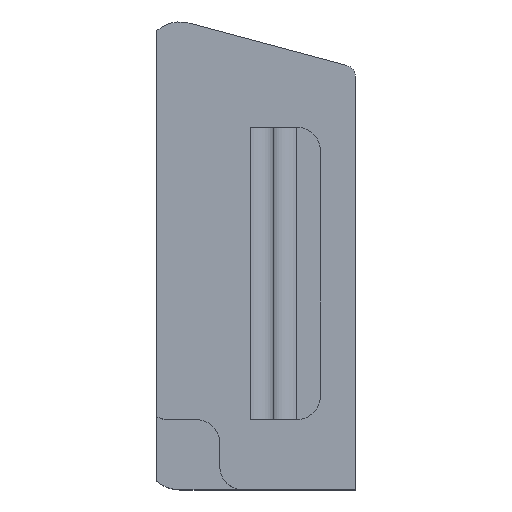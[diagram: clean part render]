
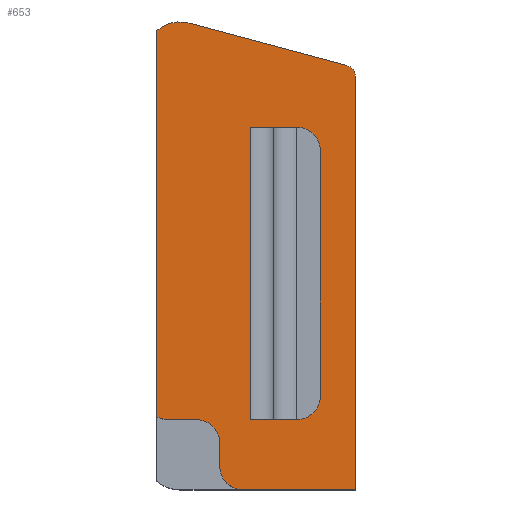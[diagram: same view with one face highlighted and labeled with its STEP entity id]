
A CAD part, top view. The second image highlights one B-rep face of the part: STEP entity #653.
In plain terms, the highlighted planar face has unit normal (0, 0, 1).
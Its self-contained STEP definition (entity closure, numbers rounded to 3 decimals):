
#122=CARTESIAN_POINT('',(-2.0,-30.732,8.0));
#123=VERTEX_POINT('',#122);
#130=CARTESIAN_POINT('',(-2.0,2.236,8.0));
#131=VERTEX_POINT('',#130);
#132=CARTESIAN_POINT('',(-2.0,2.236,8.0));
#133=DIRECTION('',(0.0,-1.0,0.0));
#134=VECTOR('',#133,32.968);
#135=LINE('',#132,#134);
#136=EDGE_CURVE('',#131,#123,#135,.T.);
#320=CARTESIAN_POINT('',(10.,-31.0,8.0));
#321=VERTEX_POINT('',#320);
#328=CARTESIAN_POINT('',(12.,-29.0,8.0));
#329=VERTEX_POINT('',#328);
#330=CARTESIAN_POINT('',(10.,-29.0,8.0));
#331=DIRECTION('',(0.0,0.0,1.0));
#332=DIRECTION('',(0.707,-0.707,0.0));
#333=AXIS2_PLACEMENT_3D('',#330,#331,#332);
#334=CIRCLE('',#333,2.0);
#335=EDGE_CURVE('',#321,#329,#334,.T.);
#361=CARTESIAN_POINT('',(6.,-31.0,8.0));
#362=VERTEX_POINT('',#361);
#370=CARTESIAN_POINT('',(10.,-31.0,8.0));
#371=DIRECTION('',(-1.0,0.0,0.0));
#372=VECTOR('',#371,4.0);
#373=LINE('',#370,#372);
#374=EDGE_CURVE('',#321,#362,#373,.T.);
#395=CARTESIAN_POINT('',(12.0,-8.0,8.0));
#396=VERTEX_POINT('',#395);
#403=CARTESIAN_POINT('',(10.0,-6.,8.0));
#404=VERTEX_POINT('',#403);
#405=CARTESIAN_POINT('',(10.0,-8.0,8.0));
#406=DIRECTION('',(0.0,0.0,1.0));
#407=DIRECTION('',(0.707,0.707,0.0));
#408=AXIS2_PLACEMENT_3D('',#405,#406,#407);
#409=CIRCLE('',#408,2.0);
#410=EDGE_CURVE('',#396,#404,#409,.T.);
#449=CARTESIAN_POINT('',(6.,-6.,8.0));
#450=VERTEX_POINT('',#449);
#451=CARTESIAN_POINT('',(10.0,-6.,8.0));
#452=DIRECTION('',(-1.0,0.0,0.0));
#453=VECTOR('',#452,4.);
#454=LINE('',#451,#453);
#455=EDGE_CURVE('',#404,#450,#454,.T.);
#489=CARTESIAN_POINT('',(6.,-6.0,8.0));
#490=DIRECTION('',(0.0,-1.0,0.0));
#491=VECTOR('',#490,25.0);
#492=LINE('',#489,#491);
#493=EDGE_CURVE('',#450,#362,#492,.T.);
#515=CARTESIAN_POINT('',(14.259,-0.715,8.0));
#516=VERTEX_POINT('',#515);
#517=CARTESIAN_POINT('',(15.,-1.681,8.0));
#518=VERTEX_POINT('',#517);
#519=CARTESIAN_POINT('',(14.,-1.681,8.0));
#520=DIRECTION('',(0.0,0.0,-1.0));
#521=DIRECTION('',(0.793,0.609,0.0));
#522=AXIS2_PLACEMENT_3D('',#519,#520,#521);
#523=CIRCLE('',#522,1.0);
#524=EDGE_CURVE('',#516,#518,#523,.T.);
#548=CARTESIAN_POINT('',(15.,-37.0,8.0));
#549=VERTEX_POINT('',#548);
#550=CARTESIAN_POINT('',(15.,-1.681,8.0));
#551=DIRECTION('',(0.0,-1.0,0.0));
#552=VECTOR('',#551,35.319);
#553=LINE('',#550,#552);
#554=EDGE_CURVE('',#518,#549,#553,.T.);
#566=CARTESIAN_POINT('',(-0.107,0.139,8.0));
#567=DIRECTION('',(0.0,0.0,1.0));
#568=DIRECTION('',(1.0,0.0,0.0));
#569=AXIS2_PLACEMENT_3D('',#566,#567,#568);
#570=PLANE('',#569);
#571=ORIENTED_EDGE('',*,*,#136,.T.);
#572=CARTESIAN_POINT('',(-1.,-31.0,8.0));
#573=VERTEX_POINT('',#572);
#574=CARTESIAN_POINT('',(-1.,-29.0,8.0));
#575=DIRECTION('',(0.0,0.0,-1.0));
#576=DIRECTION('',(-0.707,-0.707,0.0));
#577=AXIS2_PLACEMENT_3D('',#574,#575,#576);
#578=CIRCLE('',#577,2.0);
#579=EDGE_CURVE('',#573,#123,#578,.T.);
#580=ORIENTED_EDGE('',*,*,#579,.F.);
#581=CARTESIAN_POINT('',(1.4,-31.0,8.0));
#582=VERTEX_POINT('',#581);
#583=CARTESIAN_POINT('',(-1.,-31.0,8.0));
#584=DIRECTION('',(1.0,0.0,0.0));
#585=VECTOR('',#584,2.4);
#586=LINE('',#583,#585);
#587=EDGE_CURVE('',#573,#582,#586,.T.);
#588=ORIENTED_EDGE('',*,*,#587,.T.);
#589=CARTESIAN_POINT('',(3.4,-33.0,8.0));
#590=VERTEX_POINT('',#589);
#591=CARTESIAN_POINT('',(1.4,-33.0,8.0));
#592=DIRECTION('',(0.0,0.0,1.0));
#593=DIRECTION('',(0.707,0.707,0.0));
#594=AXIS2_PLACEMENT_3D('',#591,#592,#593);
#595=CIRCLE('',#594,2.0);
#596=EDGE_CURVE('',#590,#582,#595,.T.);
#597=ORIENTED_EDGE('',*,*,#596,.F.);
#598=CARTESIAN_POINT('',(3.4,-35.0,8.0));
#599=VERTEX_POINT('',#598);
#600=CARTESIAN_POINT('',(3.4,-33.0,8.0));
#601=DIRECTION('',(0.0,-1.0,0.0));
#602=VECTOR('',#601,2.0);
#603=LINE('',#600,#602);
#604=EDGE_CURVE('',#590,#599,#603,.T.);
#605=ORIENTED_EDGE('',*,*,#604,.T.);
#606=CARTESIAN_POINT('',(5.4,-37.0,8.0));
#607=VERTEX_POINT('',#606);
#608=CARTESIAN_POINT('',(5.4,-35.0,8.0));
#609=DIRECTION('',(0.0,0.0,-1.0));
#610=DIRECTION('',(-0.707,-0.707,0.0));
#611=AXIS2_PLACEMENT_3D('',#608,#609,#610);
#612=CIRCLE('',#611,2.0);
#613=EDGE_CURVE('',#607,#599,#612,.T.);
#614=ORIENTED_EDGE('',*,*,#613,.F.);
#615=CARTESIAN_POINT('',(15.,-37.0,8.0));
#616=DIRECTION('',(-1.0,0.0,0.0));
#617=VECTOR('',#616,9.6);
#618=LINE('',#615,#617);
#619=EDGE_CURVE('',#549,#607,#618,.T.);
#620=ORIENTED_EDGE('',*,*,#619,.F.);
#621=ORIENTED_EDGE('',*,*,#554,.F.);
#622=ORIENTED_EDGE('',*,*,#524,.F.);
#623=CARTESIAN_POINT('',(0.776,2.898,8.0));
#624=VERTEX_POINT('',#623);
#625=CARTESIAN_POINT('',(0.776,2.898,8.0));
#626=DIRECTION('',(0.966,-0.259,0.0));
#627=VECTOR('',#626,13.958);
#628=LINE('',#625,#627);
#629=EDGE_CURVE('',#624,#516,#628,.T.);
#630=ORIENTED_EDGE('',*,*,#629,.F.);
#631=CARTESIAN_POINT('',(0.0,0.0,8.0));
#632=DIRECTION('',(0.0,0.0,-1.0));
#633=DIRECTION('',(1.0,0.0,0.0));
#634=AXIS2_PLACEMENT_3D('',#631,#632,#633);
#635=CIRCLE('',#634,3.0);
#636=EDGE_CURVE('',#131,#624,#635,.T.);
#637=ORIENTED_EDGE('',*,*,#636,.F.);
#638=EDGE_LOOP('',(#571,#580,#588,#597,#605,#614,#620,#621,#622,#630,#637));
#639=FACE_OUTER_BOUND('',#638,.T.);
#640=CARTESIAN_POINT('',(12.,-8.0,8.0));
#641=DIRECTION('',(0.0,-1.0,0.0));
#642=VECTOR('',#641,21.0);
#643=LINE('',#640,#642);
#644=EDGE_CURVE('',#396,#329,#643,.T.);
#645=ORIENTED_EDGE('',*,*,#644,.T.);
#646=ORIENTED_EDGE('',*,*,#335,.F.);
#647=ORIENTED_EDGE('',*,*,#374,.T.);
#648=ORIENTED_EDGE('',*,*,#493,.F.);
#649=ORIENTED_EDGE('',*,*,#455,.F.);
#650=ORIENTED_EDGE('',*,*,#410,.F.);
#651=EDGE_LOOP('',(#645,#646,#647,#648,#649,#650));
#652=FACE_BOUND('',#651,.T.);
#653=ADVANCED_FACE('',(#639,#652),#570,.T.);
